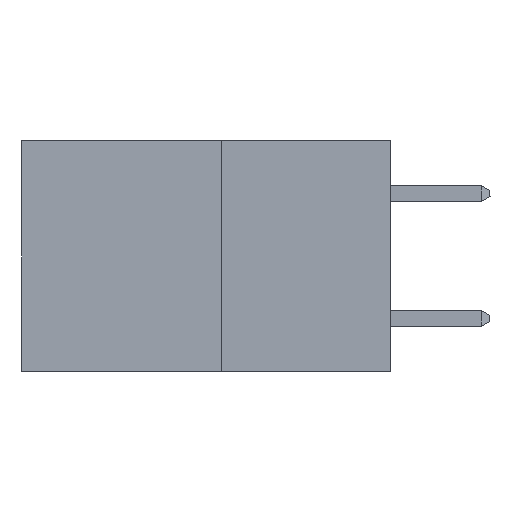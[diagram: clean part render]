
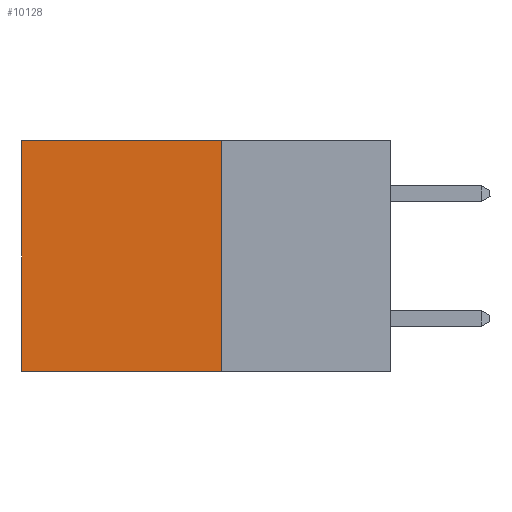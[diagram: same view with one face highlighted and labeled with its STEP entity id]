
A CAD part, left-side view. The second image highlights one B-rep face of the part: STEP entity #10128.
In plain terms, the highlighted planar face has unit normal (-1, 0, 0).
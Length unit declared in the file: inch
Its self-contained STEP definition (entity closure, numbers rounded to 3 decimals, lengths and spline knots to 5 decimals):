
#401 = VECTOR ( 'NONE', #5532, 39.37008 ) ;
#807 = EDGE_CURVE ( 'NONE', #13285, #3219, #1221, .T. ) ;
#1047 = CARTESIAN_POINT ( 'NONE',  ( 0.277, 0.27, -0.37 ) ) ;
#1221 = LINE ( 'NONE', #23560, #22210 ) ;
#1554 = VERTEX_POINT ( 'NONE', #26047 ) ;
#2189 = VECTOR ( 'NONE', #25724, 39.37008 ) ;
#3219 = VERTEX_POINT ( 'NONE', #5755 ) ;
#4387 = ORIENTED_EDGE ( 'NONE', *, *, #17101, .T. ) ;
#5042 = ORIENTED_EDGE ( 'NONE', *, *, #19175, .F. ) ;
#5532 = DIRECTION ( 'NONE',  ( 0., 0., -1. ) ) ;
#5755 = CARTESIAN_POINT ( 'NONE',  ( 0.277, 0.59, -0.37 ) ) ;
#5785 = PLANE ( 'NONE',  #16408 ) ;
#7935 = DIRECTION ( 'NONE',  ( 0., 0., -1. ) ) ;
#8660 = DIRECTION ( 'NONE',  ( 0., 1., 0. ) ) ;
#9038 = CARTESIAN_POINT ( 'NONE',  ( 0.277, 0.59, -0.37 ) ) ;
#9200 = FACE_OUTER_BOUND ( 'NONE', #27060, .T. ) ;
#9928 = VERTEX_POINT ( 'NONE', #15718 ) ;
#10128 = ADVANCED_FACE ( 'NONE', ( #9200 ), #5785, .F. ) ;
#10471 = VECTOR ( 'NONE', #8660, 39.37008 ) ;
#12016 = CARTESIAN_POINT ( 'NONE',  ( 0.277, 0.27, -0.37 ) ) ;
#13285 = VERTEX_POINT ( 'NONE', #1047 ) ;
#15718 = CARTESIAN_POINT ( 'NONE',  ( 0.277, 0.27, 0. ) ) ;
#16408 = AXIS2_PLACEMENT_3D ( 'NONE', #12016, #20399, #7935 ) ;
#17101 = EDGE_CURVE ( 'NONE', #1554, #3219, #25776, .T. ) ;
#19175 = EDGE_CURVE ( 'NONE', #9928, #13285, #23370, .T. ) ;
#20399 = DIRECTION ( 'NONE',  ( 1., 0., 0. ) ) ;
#20552 = ORIENTED_EDGE ( 'NONE', *, *, #24108, .T. ) ;
#20885 = LINE ( 'NONE', #21134, #10471 ) ;
#21134 = CARTESIAN_POINT ( 'NONE',  ( 0.277, 0.27, 0. ) ) ;
#22210 = VECTOR ( 'NONE', #24217, 39.37008 ) ;
#23370 = LINE ( 'NONE', #24371, #401 ) ;
#23560 = CARTESIAN_POINT ( 'NONE',  ( 0.277, 0.27, -0.37 ) ) ;
#24108 = EDGE_CURVE ( 'NONE', #9928, #1554, #20885, .T. ) ;
#24217 = DIRECTION ( 'NONE',  ( 0., 1., 0. ) ) ;
#24371 = CARTESIAN_POINT ( 'NONE',  ( 0.277, 0.27, -0.37 ) ) ;
#24756 = ORIENTED_EDGE ( 'NONE', *, *, #807, .F. ) ;
#25724 = DIRECTION ( 'NONE',  ( 0., 0., -1. ) ) ;
#25776 = LINE ( 'NONE', #9038, #2189 ) ;
#26047 = CARTESIAN_POINT ( 'NONE',  ( 0.277, 0.59, 0. ) ) ;
#27060 = EDGE_LOOP ( 'NONE', ( #4387, #24756, #5042, #20552 ) ) ;
